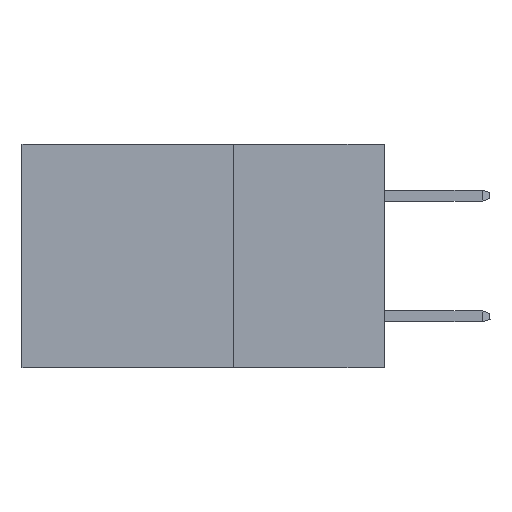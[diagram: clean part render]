
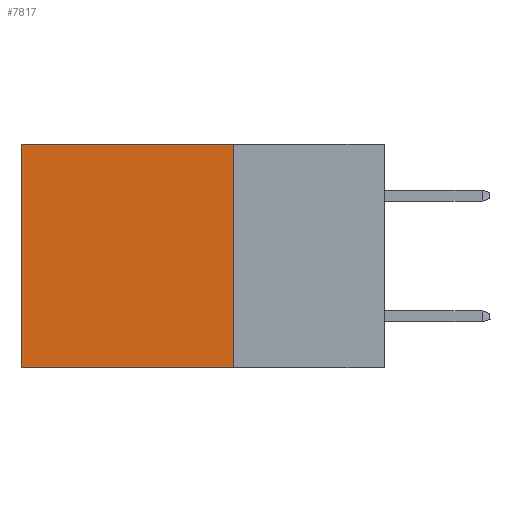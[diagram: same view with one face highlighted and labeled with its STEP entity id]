
A CAD part, left-side view. The second image highlights one B-rep face of the part: STEP entity #7817.
In plain terms, the highlighted planar face has unit normal (-1, 0, 0).
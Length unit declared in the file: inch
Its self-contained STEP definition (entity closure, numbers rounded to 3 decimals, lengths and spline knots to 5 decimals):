
#294 = PLANE ( 'NONE',  #9542 ) ;
#447 = LINE ( 'NONE', #4127, #7930 ) ;
#564 = DIRECTION ( 'NONE',  ( 0., 0., -1. ) ) ;
#841 = EDGE_CURVE ( 'NONE', #8793, #2461, #4438, .T. ) ;
#1562 = VERTEX_POINT ( 'NONE', #6111 ) ;
#1738 = ORIENTED_EDGE ( 'NONE', *, *, #7106, .T. ) ;
#1839 = DIRECTION ( 'NONE',  ( 0., 0., -1. ) ) ;
#2110 = DIRECTION ( 'NONE',  ( 0., 1., 0. ) ) ;
#2162 = DIRECTION ( 'NONE',  ( 1., 0., 0. ) ) ;
#2461 = VERTEX_POINT ( 'NONE', #4880 ) ;
#2730 = CARTESIAN_POINT ( 'NONE',  ( 0.2615, 0.6, -0.37 ) ) ;
#2793 = DIRECTION ( 'NONE',  ( 0., 1., 0. ) ) ;
#3502 = VECTOR ( 'NONE', #2110, 39.37008 ) ;
#3963 = VECTOR ( 'NONE', #8217, 39.37008 ) ;
#4127 = CARTESIAN_POINT ( 'NONE',  ( 0.2615, 0.25, -0.37 ) ) ;
#4167 = EDGE_CURVE ( 'NONE', #6097, #2461, #10018, .T. ) ;
#4438 = LINE ( 'NONE', #2730, #3963 ) ;
#4880 = CARTESIAN_POINT ( 'NONE',  ( 0.2615, 0.6, -0.37 ) ) ;
#5131 = ORIENTED_EDGE ( 'NONE', *, *, #841, .T. ) ;
#5336 = CARTESIAN_POINT ( 'NONE',  ( 0.2615, 0.6, 0. ) ) ;
#6086 = CARTESIAN_POINT ( 'NONE',  ( 0.2615, 0.25, -0.37 ) ) ;
#6097 = VERTEX_POINT ( 'NONE', #6086 ) ;
#6111 = CARTESIAN_POINT ( 'NONE',  ( 0.2615, 0.25, 0. ) ) ;
#6470 = VECTOR ( 'NONE', #2793, 39.37008 ) ;
#6500 = CARTESIAN_POINT ( 'NONE',  ( 0.2615, 0.25, -0.37 ) ) ;
#7106 = EDGE_CURVE ( 'NONE', #1562, #8793, #9787, .T. ) ;
#7459 = CARTESIAN_POINT ( 'NONE',  ( 0.2615, 0.25, -0.37 ) ) ;
#7817 = ADVANCED_FACE ( 'NONE', ( #8670 ), #294, .F. ) ;
#7930 = VECTOR ( 'NONE', #1839, 39.37008 ) ;
#8217 = DIRECTION ( 'NONE',  ( 0., 0., -1. ) ) ;
#8463 = CARTESIAN_POINT ( 'NONE',  ( 0.2615, 0.25, 0. ) ) ;
#8670 = FACE_OUTER_BOUND ( 'NONE', #9618, .T. ) ;
#8727 = EDGE_CURVE ( 'NONE', #1562, #6097, #447, .T. ) ;
#8793 = VERTEX_POINT ( 'NONE', #5336 ) ;
#9542 = AXIS2_PLACEMENT_3D ( 'NONE', #6500, #2162, #564 ) ;
#9618 = EDGE_LOOP ( 'NONE', ( #5131, #10110, #10041, #1738 ) ) ;
#9787 = LINE ( 'NONE', #8463, #3502 ) ;
#10018 = LINE ( 'NONE', #7459, #6470 ) ;
#10041 = ORIENTED_EDGE ( 'NONE', *, *, #8727, .F. ) ;
#10110 = ORIENTED_EDGE ( 'NONE', *, *, #4167, .F. ) ;
